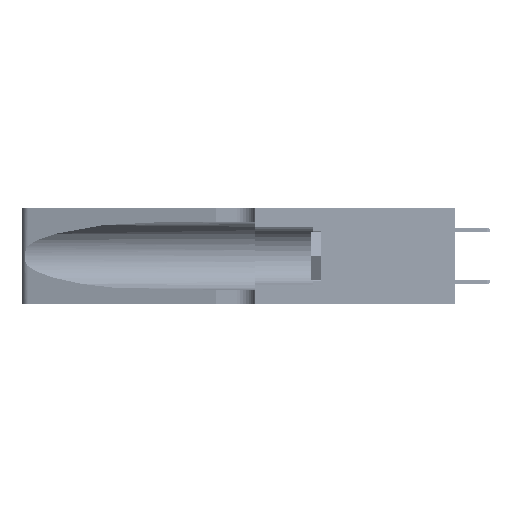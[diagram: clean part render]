
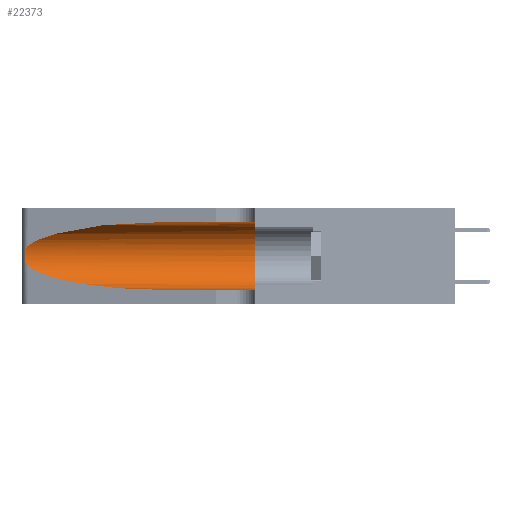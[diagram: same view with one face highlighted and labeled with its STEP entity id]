
A CAD part, left-side view. The second image highlights one B-rep face of the part: STEP entity #22373.
In plain terms, the highlighted cylindrical face has radius 3.308 mm (diameter 6.617 mm), a partial arc.
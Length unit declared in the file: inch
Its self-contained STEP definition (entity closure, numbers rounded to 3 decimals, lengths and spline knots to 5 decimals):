
#765 = VERTEX_POINT ( 'NONE', #6537 ) ;
#909 = CARTESIAN_POINT ( 'NONE',  ( 0.25639, 1.23184, 0.21858 ) ) ;
#2159 = VECTOR ( 'NONE', #4079, 39.37008 ) ;
#2239 =( BOUNDED_CURVE ( )  B_SPLINE_CURVE ( 3, ( #46356, #11936, #30787, #27263 ),
 .UNSPECIFIED., .F., .F. ) 
 B_SPLINE_CURVE_WITH_KNOTS ( ( 4, 4 ),
 ( 1.5708, 2.84003 ),
 .UNSPECIFIED. ) 
 CURVE ( )  GEOMETRIC_REPRESENTATION_ITEM ( )  RATIONAL_B_SPLINE_CURVE ( ( 1., 0.87, 0.87, 1. ) ) 
 REPRESENTATION_ITEM ( '' )  );
#2488 = CARTESIAN_POINT ( 'NONE',  ( 0.25487, 1.22718, 0.14631 ) ) ;
#3579 = DIRECTION ( 'NONE',  ( 0., 0., 1. ) ) ;
#4079 = DIRECTION ( 'NONE',  ( 0., -1., 0. ) ) ;
#5786 = AXIS2_PLACEMENT_3D ( 'NONE', #37345, #10974, #6945 ) ;
#5838 = ORIENTED_EDGE ( 'NONE', *, *, #13194, .T. ) ;
#6537 = CARTESIAN_POINT ( 'NONE',  ( 0.1305, 0.72297, 0.05475 ) ) ;
#6945 = DIRECTION ( 'NONE',  ( 0., 0., -1. ) ) ;
#7145 = EDGE_CURVE ( 'NONE', #29096, #26855, #25559, .T. ) ;
#7690 = CYLINDRICAL_SURFACE ( 'NONE', #5786, 0.13025 ) ;
#8903 = CIRCLE ( 'NONE', #38572, 0.13025 ) ;
#9484 = CARTESIAN_POINT ( 'NONE',  ( 0.25789, 1.23486, 0.15765 ) ) ;
#10974 = DIRECTION ( 'NONE',  ( 0., -1., 0. ) ) ;
#11766 = CARTESIAN_POINT ( 'NONE',  ( 0.25487, 1.22718, 0.22369 ) ) ;
#11936 = CARTESIAN_POINT ( 'NONE',  ( 0.18966, 0.96281, 0.31525 ) ) ;
#13194 = EDGE_CURVE ( 'NONE', #26855, #765, #35006, .T. ) ;
#16263 = CARTESIAN_POINT ( 'NONE',  ( 0.25787, 1.23484, 0.2124 ) ) ;
#17007 = CARTESIAN_POINT ( 'NONE',  ( 0.25487, 1.22718, 0.14631 ) ) ;
#17252 = CARTESIAN_POINT ( 'NONE',  ( 0.25856, 1.23593, 0.16098 ) ) ;
#19007 = CARTESIAN_POINT ( 'NONE',  ( 0.25487, 1.22718, 0.22369 ) ) ;
#20172 = CARTESIAN_POINT ( 'NONE',  ( 0.1305, 1.61858, 0.05475 ) ) ;
#20208 = VERTEX_POINT ( 'NONE', #24353 ) ;
#21265 = CARTESIAN_POINT ( 'NONE',  ( 0.1305, 0.35, 0.31525 ) ) ;
#21475 = ORIENTED_EDGE ( 'NONE', *, *, #31545, .T. ) ;
#22373 = ADVANCED_FACE ( 'NONE', ( #45124 ), #7690, .F. ) ;
#22395 = CARTESIAN_POINT ( 'NONE',  ( 0.25487, 1.22718, 0.14631 ) ) ;
#23759 = ORIENTED_EDGE ( 'NONE', *, *, #7145, .T. ) ;
#24353 = CARTESIAN_POINT ( 'NONE',  ( 0.1305, 0.72297, 0.31525 ) ) ;
#25054 = VERTEX_POINT ( 'NONE', #26112 ) ;
#25559 = B_SPLINE_CURVE_WITH_KNOTS ( 'NONE', 3,
 ( #11766, #27084, #909, #16263, #42391, #27840, #46925, #43154, #44126, #17252, #9484, #48138, #28080, #17007 ),
 .UNSPECIFIED., .F., .F.,
 ( 4, 2, 2, 2, 2, 2, 4 ),
 ( 0., 0.00027, 0.00053, 0.00107, 0.0016, 0.00187, 0.00214 ),
 .UNSPECIFIED. ) ;
#25963 = CARTESIAN_POINT ( 'NONE',  ( 0.1305, 1.61858, 0.31525 ) ) ;
#26112 = CARTESIAN_POINT ( 'NONE',  ( 0.1305, 0.35, 0.05475 ) ) ;
#26711 = DIRECTION ( 'NONE',  ( 0., 1., 0. ) ) ;
#26855 = VERTEX_POINT ( 'NONE', #22395 ) ;
#27084 = CARTESIAN_POINT ( 'NONE',  ( 0.25555, 1.22994, 0.2215 ) ) ;
#27263 = CARTESIAN_POINT ( 'NONE',  ( 0.25487, 1.22718, 0.22369 ) ) ;
#27840 = CARTESIAN_POINT ( 'NONE',  ( 0.26018, 1.23835, 0.19895 ) ) ;
#28080 = CARTESIAN_POINT ( 'NONE',  ( 0.25555, 1.22993, 0.14849 ) ) ;
#29096 = VERTEX_POINT ( 'NONE', #19007 ) ;
#29410 = CARTESIAN_POINT ( 'NONE',  ( 0.1305, 0.72297, 0.05475 ) ) ;
#30695 = EDGE_CURVE ( 'NONE', #20208, #40507, #45048, .T. ) ;
#30787 = CARTESIAN_POINT ( 'NONE',  ( 0.2373, 1.15595, 0.28018 ) ) ;
#31545 = EDGE_CURVE ( 'NONE', #765, #25054, #31742, .T. ) ;
#31742 = LINE ( 'NONE', #20172, #44776 ) ;
#32162 = ORIENTED_EDGE ( 'NONE', *, *, #36812, .F. ) ;
#35006 =( BOUNDED_CURVE ( )  B_SPLINE_CURVE ( 3, ( #2488, #45211, #37431, #29410 ),
 .UNSPECIFIED., .F., .F. ) 
 B_SPLINE_CURVE_WITH_KNOTS ( ( 4, 4 ),
 ( 3.44316, 4.71239 ),
 .UNSPECIFIED. ) 
 CURVE ( )  GEOMETRIC_REPRESENTATION_ITEM ( )  RATIONAL_B_SPLINE_CURVE ( ( 1., 0.87, 0.87, 1. ) ) 
 REPRESENTATION_ITEM ( '' )  );
#36812 = EDGE_CURVE ( 'NONE', #40507, #25054, #8903, .T. ) ;
#37345 = CARTESIAN_POINT ( 'NONE',  ( 0.1305, 1.61858, 0.185 ) ) ;
#37431 = CARTESIAN_POINT ( 'NONE',  ( 0.18966, 0.96281, 0.05475 ) ) ;
#38005 = CARTESIAN_POINT ( 'NONE',  ( 0.1305, 0.35, 0.185 ) ) ;
#38572 = AXIS2_PLACEMENT_3D ( 'NONE', #38005, #26711, #3579 ) ;
#39200 = ORIENTED_EDGE ( 'NONE', *, *, #42196, .T. ) ;
#39248 = DIRECTION ( 'NONE',  ( 0., -1., 0. ) ) ;
#40507 = VERTEX_POINT ( 'NONE', #21265 ) ;
#41923 = EDGE_LOOP ( 'NONE', ( #39200, #23759, #5838, #21475, #32162, #48979 ) ) ;
#42196 = EDGE_CURVE ( 'NONE', #20208, #29096, #2239, .T. ) ;
#42391 = CARTESIAN_POINT ( 'NONE',  ( 0.25854, 1.2359, 0.20912 ) ) ;
#43154 = CARTESIAN_POINT ( 'NONE',  ( 0.26075, 1.23896, 0.178 ) ) ;
#44126 = CARTESIAN_POINT ( 'NONE',  ( 0.26017, 1.23833, 0.17102 ) ) ;
#44776 = VECTOR ( 'NONE', #39248, 39.37008 ) ;
#45048 = LINE ( 'NONE', #25963, #2159 ) ;
#45124 = FACE_OUTER_BOUND ( 'NONE', #41923, .T. ) ;
#45211 = CARTESIAN_POINT ( 'NONE',  ( 0.2373, 1.15595, 0.08982 ) ) ;
#46356 = CARTESIAN_POINT ( 'NONE',  ( 0.1305, 0.72297, 0.31525 ) ) ;
#46925 = CARTESIAN_POINT ( 'NONE',  ( 0.26075, 1.23896, 0.19203 ) ) ;
#48138 = CARTESIAN_POINT ( 'NONE',  ( 0.25639, 1.23186, 0.15144 ) ) ;
#48979 = ORIENTED_EDGE ( 'NONE', *, *, #30695, .F. ) ;
